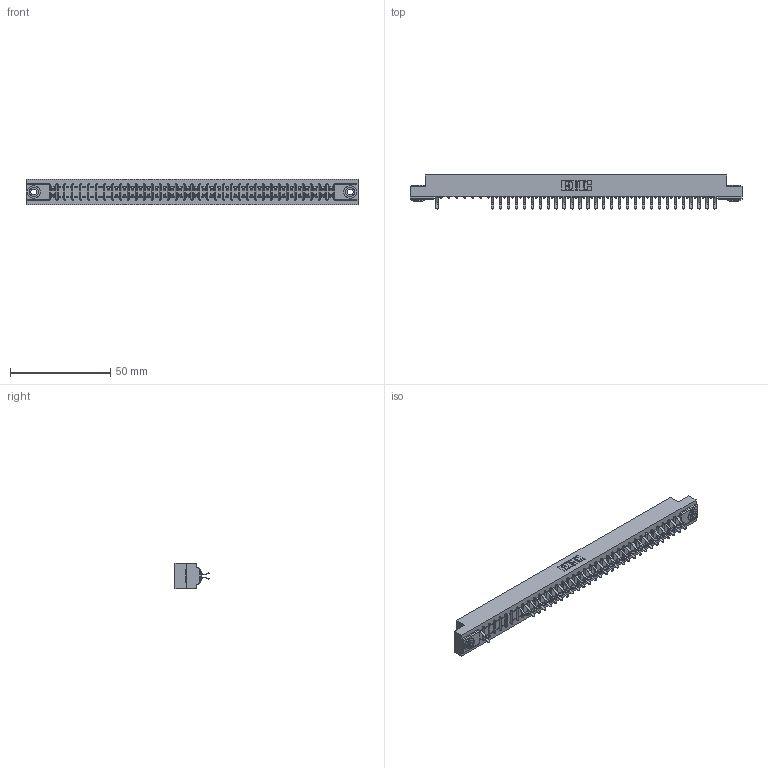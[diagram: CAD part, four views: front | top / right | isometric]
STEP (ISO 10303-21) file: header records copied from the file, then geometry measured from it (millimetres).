
FILE_DESCRIPTION (( 'STEP AP203' ), '1' );
FILE_NAME ('307-072-556-203.STEP', '2018-08-06T15:39:04', ( '' ), ( '' ), 'SwSTEP 2.0', 'SolidWorks 2016', '' );
FILE_SCHEMA (( 'CONFIG_CONTROL_DESIGN' ));
Length unit declared in the file: inch
Products named in the file (4): 307 Part_.156 Dia Mounting Holes; 307-290-001_556; 345-250-002_345-250-002-102; 307-072-556-203
Assembly tree (62 placements, depth 2):
  307-072-556-203
    307 Part_.156 Dia Mounting Holes
    307-290-001_556  x59
    345-250-002_345-250-002-102  x2
Bounding box: 165.66 x 16.97 x 12.7 mm (x, y, z)
Volume: 17395.6 mm3; surface area: 20153.2 mm2
Topology: 62 solids, 62 shells, 3287 faces, 9229 edges, 5970 vertices
Faces by surface type: plane 2119, cylinder 1086, sphere 74, cone 8
Entity records: 33507 total; most frequent: CARTESIAN_POINT 5520, ORIENTED_EDGE 5474, DIRECTION 5411, EDGE_CURVE 2737, VECTOR 2089, LINE 2089, VERTEX_POINT 1770, AXIS2_PLACEMENT_3D 1661
